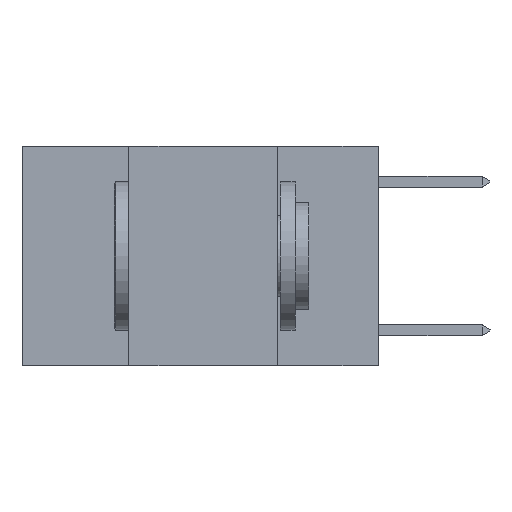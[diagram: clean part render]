
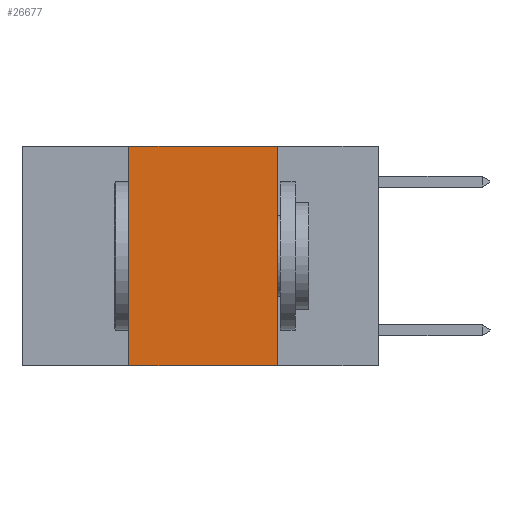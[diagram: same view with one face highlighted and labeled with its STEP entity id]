
A CAD part, left-side view. The second image highlights one B-rep face of the part: STEP entity #26677.
In plain terms, the highlighted planar face has unit normal (-1, 0, 0).
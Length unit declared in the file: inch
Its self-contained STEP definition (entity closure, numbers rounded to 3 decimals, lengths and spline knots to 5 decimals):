
#43 = CARTESIAN_POINT ( 'NONE',  ( 0., 0.42, 0. ) ) ;
#1914 = DIRECTION ( 'NONE',  ( 0., 0., -1. ) ) ;
#2714 = DIRECTION ( 'NONE',  ( 0., -1., 0. ) ) ;
#4069 = ORIENTED_EDGE ( 'NONE', *, *, #17055, .T. ) ;
#4087 = ORIENTED_EDGE ( 'NONE', *, *, #7237, .F. ) ;
#4165 = CARTESIAN_POINT ( 'NONE',  ( 0., 0.6, 0. ) ) ;
#5867 = PLANE ( 'NONE',  #25692 ) ;
#6502 = LINE ( 'NONE', #15073, #12892 ) ;
#6659 = VERTEX_POINT ( 'NONE', #21339 ) ;
#7237 = EDGE_CURVE ( 'NONE', #15348, #6659, #8932, .T. ) ;
#7743 = DIRECTION ( 'NONE',  ( 0., -1., 0. ) ) ;
#8932 = LINE ( 'NONE', #19775, #12950 ) ;
#9819 = LINE ( 'NONE', #26995, #15108 ) ;
#10372 = EDGE_CURVE ( 'NONE', #26304, #21918, #13521, .T. ) ;
#12363 = EDGE_CURVE ( 'NONE', #21918, #15348, #9819, .T. ) ;
#12385 = ORIENTED_EDGE ( 'NONE', *, *, #10372, .F. ) ;
#12468 = CARTESIAN_POINT ( 'NONE',  ( 0., 0.42, -0.37 ) ) ;
#12892 = VECTOR ( 'NONE', #2714, 39.37008 ) ;
#12950 = VECTOR ( 'NONE', #17777, 39.37008 ) ;
#13521 = LINE ( 'NONE', #15509, #26059 ) ;
#15073 = CARTESIAN_POINT ( 'NONE',  ( 0., 0.6, -0.37 ) ) ;
#15108 = VECTOR ( 'NONE', #7743, 39.37008 ) ;
#15348 = VERTEX_POINT ( 'NONE', #20832 ) ;
#15509 = CARTESIAN_POINT ( 'NONE',  ( 0., 0.42, 0. ) ) ;
#17055 = EDGE_CURVE ( 'NONE', #26304, #6659, #6502, .T. ) ;
#17345 = ORIENTED_EDGE ( 'NONE', *, *, #12363, .F. ) ;
#17777 = DIRECTION ( 'NONE',  ( 0., 0., -1. ) ) ;
#17880 = DIRECTION ( 'NONE',  ( 0., 0., 1. ) ) ;
#18623 = DIRECTION ( 'NONE',  ( 1., 0., 0. ) ) ;
#19775 = CARTESIAN_POINT ( 'NONE',  ( 0., 0.17, 0. ) ) ;
#20832 = CARTESIAN_POINT ( 'NONE',  ( 0., 0.17, 0. ) ) ;
#21339 = CARTESIAN_POINT ( 'NONE',  ( 0., 0.17, -0.37 ) ) ;
#21918 = VERTEX_POINT ( 'NONE', #43 ) ;
#23416 = FACE_OUTER_BOUND ( 'NONE', #26279, .T. ) ;
#25692 = AXIS2_PLACEMENT_3D ( 'NONE', #4165, #18623, #1914 ) ;
#26059 = VECTOR ( 'NONE', #17880, 39.37008 ) ;
#26279 = EDGE_LOOP ( 'NONE', ( #4087, #17345, #12385, #4069 ) ) ;
#26304 = VERTEX_POINT ( 'NONE', #12468 ) ;
#26677 = ADVANCED_FACE ( 'NONE', ( #23416 ), #5867, .F. ) ;
#26995 = CARTESIAN_POINT ( 'NONE',  ( 0., 0.6, 0. ) ) ;
